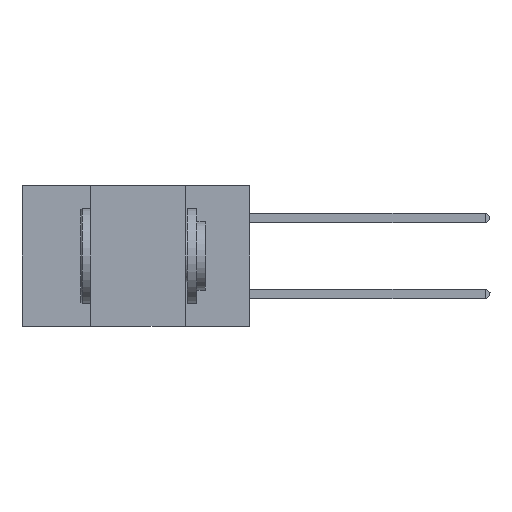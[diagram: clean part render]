
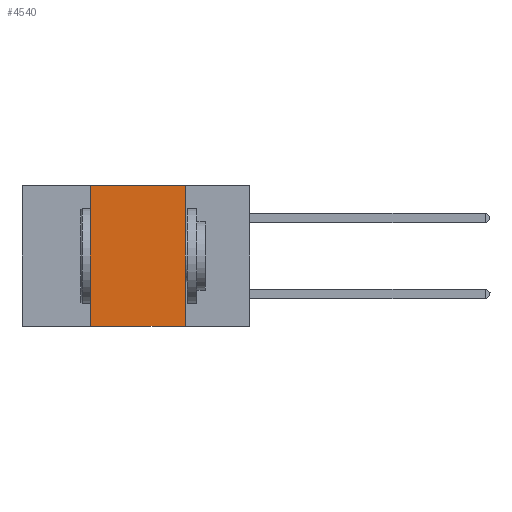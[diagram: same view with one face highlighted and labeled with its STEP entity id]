
A CAD part, left-side view. The second image highlights one B-rep face of the part: STEP entity #4540.
In plain terms, the highlighted planar face has unit normal (-1, 0, 0).
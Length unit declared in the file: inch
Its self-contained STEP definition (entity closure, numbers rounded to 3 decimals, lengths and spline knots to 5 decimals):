
#51 = EDGE_CURVE ( 'NONE', #11812, #6402, #8423, .T. ) ;
#680 = CARTESIAN_POINT ( 'NONE',  ( 0., 0.6, 0. ) ) ;
#1173 = VECTOR ( 'NONE', #3454, 39.37008 ) ;
#1228 = AXIS2_PLACEMENT_3D ( 'NONE', #4176, #4568, #4523 ) ;
#1338 = VERTEX_POINT ( 'NONE', #5466 ) ;
#2072 = CARTESIAN_POINT ( 'NONE',  ( 0., 0.42, -0.37 ) ) ;
#2273 = ORIENTED_EDGE ( 'NONE', *, *, #3808, .F. ) ;
#2344 = CARTESIAN_POINT ( 'NONE',  ( 0., 0.17, 0. ) ) ;
#3454 = DIRECTION ( 'NONE',  ( 0., 0., -1. ) ) ;
#3699 = CARTESIAN_POINT ( 'NONE',  ( 0., 0.42, 0. ) ) ;
#3715 = DIRECTION ( 'NONE',  ( 0., 0., 1. ) ) ;
#3793 = PLANE ( 'NONE',  #1228 ) ;
#3808 = EDGE_CURVE ( 'NONE', #11812, #1338, #8201, .T. ) ;
#4022 = DIRECTION ( 'NONE',  ( 0., -1., 0. ) ) ;
#4176 = CARTESIAN_POINT ( 'NONE',  ( 0., 0.6, 0. ) ) ;
#4523 = DIRECTION ( 'NONE',  ( 0., 0., -1. ) ) ;
#4540 = ADVANCED_FACE ( 'NONE', ( #12836 ), #3793, .F. ) ;
#4568 = DIRECTION ( 'NONE',  ( 1., 0., 0. ) ) ;
#4783 = ORIENTED_EDGE ( 'NONE', *, *, #6252, .F. ) ;
#5136 = ORIENTED_EDGE ( 'NONE', *, *, #51, .T. ) ;
#5222 = EDGE_CURVE ( 'NONE', #10104, #6402, #12026, .T. ) ;
#5466 = CARTESIAN_POINT ( 'NONE',  ( 0., 0.42, 0. ) ) ;
#6252 = EDGE_CURVE ( 'NONE', #1338, #10104, #10405, .T. ) ;
#6402 = VERTEX_POINT ( 'NONE', #11488 ) ;
#7394 = CARTESIAN_POINT ( 'NONE',  ( 0., 0.6, -0.37 ) ) ;
#7878 = VECTOR ( 'NONE', #3715, 39.37008 ) ;
#8201 = LINE ( 'NONE', #3699, #7878 ) ;
#8216 = DIRECTION ( 'NONE',  ( 0., -1., 0. ) ) ;
#8423 = LINE ( 'NONE', #7394, #10867 ) ;
#9147 = EDGE_LOOP ( 'NONE', ( #12700, #4783, #2273, #5136 ) ) ;
#9296 = CARTESIAN_POINT ( 'NONE',  ( 0., 0.17, 0. ) ) ;
#10104 = VERTEX_POINT ( 'NONE', #9296 ) ;
#10405 = LINE ( 'NONE', #680, #12792 ) ;
#10867 = VECTOR ( 'NONE', #8216, 39.37008 ) ;
#11488 = CARTESIAN_POINT ( 'NONE',  ( 0., 0.17, -0.37 ) ) ;
#11812 = VERTEX_POINT ( 'NONE', #2072 ) ;
#12026 = LINE ( 'NONE', #2344, #1173 ) ;
#12700 = ORIENTED_EDGE ( 'NONE', *, *, #5222, .F. ) ;
#12792 = VECTOR ( 'NONE', #4022, 39.37008 ) ;
#12836 = FACE_OUTER_BOUND ( 'NONE', #9147, .T. ) ;
